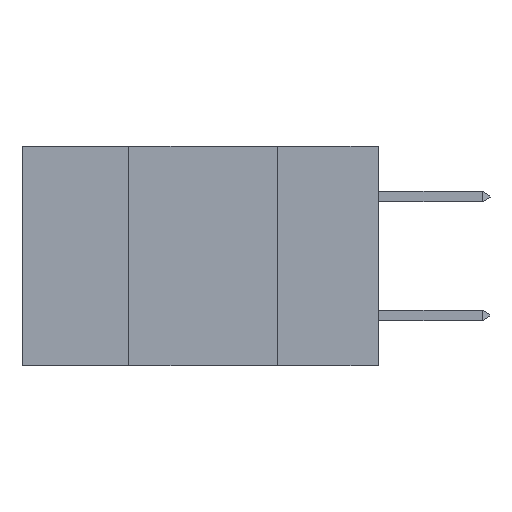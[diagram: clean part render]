
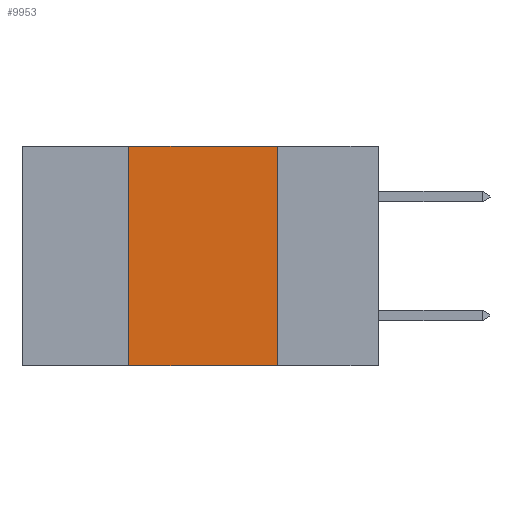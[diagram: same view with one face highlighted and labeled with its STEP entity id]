
A CAD part, left-side view. The second image highlights one B-rep face of the part: STEP entity #9953.
In plain terms, the highlighted planar face has unit normal (-1, 0, 0).
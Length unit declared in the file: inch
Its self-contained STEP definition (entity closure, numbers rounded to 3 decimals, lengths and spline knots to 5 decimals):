
#1876 = ORIENTED_EDGE ( 'NONE', *, *, #6875, .T. ) ;
#3972 = PLANE ( 'NONE',  #14083 ) ;
#4406 = CARTESIAN_POINT ( 'NONE',  ( 0., 0.17, 0. ) ) ;
#6364 = DIRECTION ( 'NONE',  ( 0., 0., -1. ) ) ;
#6875 = EDGE_CURVE ( 'NONE', #29695, #13326, #20480, .T. ) ;
#7013 = VERTEX_POINT ( 'NONE', #21444 ) ;
#7026 = CARTESIAN_POINT ( 'NONE',  ( 0., 0.6, -0.37 ) ) ;
#7076 = VECTOR ( 'NONE', #12807, 39.37008 ) ;
#7094 = EDGE_LOOP ( 'NONE', ( #15991, #14007, #25771, #1876 ) ) ;
#7539 = EDGE_CURVE ( 'NONE', #7013, #19599, #13396, .T. ) ;
#9953 = ADVANCED_FACE ( 'NONE', ( #25946 ), #3972, .F. ) ;
#11010 = CARTESIAN_POINT ( 'NONE',  ( 0., 0.17, 0. ) ) ;
#11231 = CARTESIAN_POINT ( 'NONE',  ( 0., 0.6, 0. ) ) ;
#11689 = DIRECTION ( 'NONE',  ( 0., -1., 0. ) ) ;
#12718 = CARTESIAN_POINT ( 'NONE',  ( 0., 0.6, 0. ) ) ;
#12807 = DIRECTION ( 'NONE',  ( 0., 0., 1. ) ) ;
#13228 = CARTESIAN_POINT ( 'NONE',  ( 0., 0.42, 0. ) ) ;
#13326 = VERTEX_POINT ( 'NONE', #30671 ) ;
#13396 = LINE ( 'NONE', #12718, #27905 ) ;
#14007 = ORIENTED_EDGE ( 'NONE', *, *, #7539, .F. ) ;
#14083 = AXIS2_PLACEMENT_3D ( 'NONE', #11231, #25801, #6364 ) ;
#15991 = ORIENTED_EDGE ( 'NONE', *, *, #20275, .F. ) ;
#18823 = DIRECTION ( 'NONE',  ( 0., 0., -1. ) ) ;
#19044 = VECTOR ( 'NONE', #18823, 39.37008 ) ;
#19317 = CARTESIAN_POINT ( 'NONE',  ( 0., 0.42, -0.37 ) ) ;
#19599 = VERTEX_POINT ( 'NONE', #11010 ) ;
#20275 = EDGE_CURVE ( 'NONE', #19599, #13326, #26147, .T. ) ;
#20480 = LINE ( 'NONE', #7026, #27231 ) ;
#21444 = CARTESIAN_POINT ( 'NONE',  ( 0., 0.42, 0. ) ) ;
#24781 = DIRECTION ( 'NONE',  ( 0., -1., 0. ) ) ;
#25771 = ORIENTED_EDGE ( 'NONE', *, *, #27632, .F. ) ;
#25801 = DIRECTION ( 'NONE',  ( 1., 0., 0. ) ) ;
#25946 = FACE_OUTER_BOUND ( 'NONE', #7094, .T. ) ;
#26147 = LINE ( 'NONE', #4406, #19044 ) ;
#27231 = VECTOR ( 'NONE', #11689, 39.37008 ) ;
#27632 = EDGE_CURVE ( 'NONE', #29695, #7013, #29038, .T. ) ;
#27905 = VECTOR ( 'NONE', #24781, 39.37008 ) ;
#29038 = LINE ( 'NONE', #13228, #7076 ) ;
#29695 = VERTEX_POINT ( 'NONE', #19317 ) ;
#30671 = CARTESIAN_POINT ( 'NONE',  ( 0., 0.17, -0.37 ) ) ;
